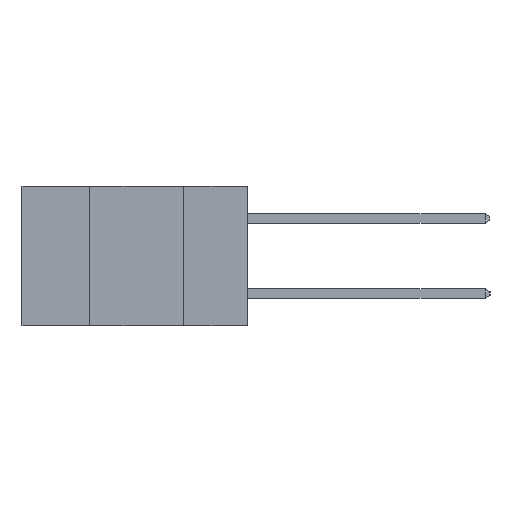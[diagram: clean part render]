
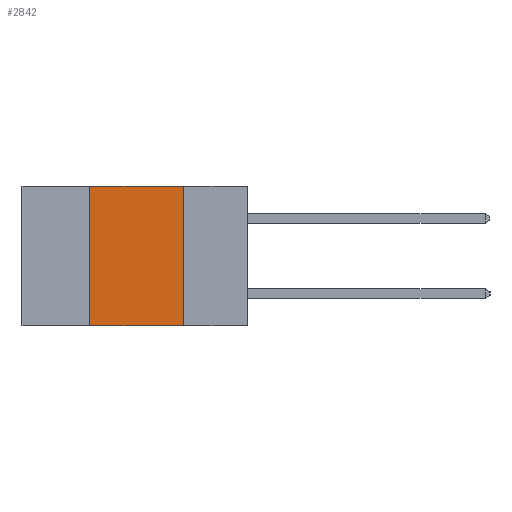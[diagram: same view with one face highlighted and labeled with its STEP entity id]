
A CAD part, left-side view. The second image highlights one B-rep face of the part: STEP entity #2842.
In plain terms, the highlighted planar face has unit normal (-1, 0, 0).
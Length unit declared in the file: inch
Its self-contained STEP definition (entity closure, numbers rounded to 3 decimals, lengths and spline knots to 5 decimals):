
#142 = VECTOR ( 'NONE', #5991, 39.37008 ) ;
#440 = VECTOR ( 'NONE', #12052, 39.37008 ) ;
#1023 = VERTEX_POINT ( 'NONE', #17797 ) ;
#1209 = DIRECTION ( 'NONE',  ( 0., 0., -1. ) ) ;
#1297 = ORIENTED_EDGE ( 'NONE', *, *, #7673, .F. ) ;
#1351 = DIRECTION ( 'NONE',  ( 1., 0., 0. ) ) ;
#1545 = CARTESIAN_POINT ( 'NONE',  ( 0., 0.6, 0. ) ) ;
#1563 = PLANE ( 'NONE',  #12263 ) ;
#1833 = DIRECTION ( 'NONE',  ( 0., 0., 1. ) ) ;
#2842 = ADVANCED_FACE ( 'NONE', ( #9797 ), #1563, .F. ) ;
#2992 = VERTEX_POINT ( 'NONE', #19221 ) ;
#3290 = CARTESIAN_POINT ( 'NONE',  ( 0., 0.42, -0.37 ) ) ;
#3677 = DIRECTION ( 'NONE',  ( 0., 0., -1. ) ) ;
#4382 = EDGE_CURVE ( 'NONE', #12080, #2992, #7931, .T. ) ;
#5432 = CARTESIAN_POINT ( 'NONE',  ( 0., 0.17, -0.37 ) ) ;
#5991 = DIRECTION ( 'NONE',  ( 0., -1., 0. ) ) ;
#6108 = CARTESIAN_POINT ( 'NONE',  ( 0., 0.6, -0.37 ) ) ;
#7249 = LINE ( 'NONE', #19880, #20159 ) ;
#7673 = EDGE_CURVE ( 'NONE', #2992, #1023, #9186, .T. ) ;
#7931 = LINE ( 'NONE', #3290, #19820 ) ;
#9010 = ORIENTED_EDGE ( 'NONE', *, *, #20681, .F. ) ;
#9186 = LINE ( 'NONE', #12073, #440 ) ;
#9338 = ORIENTED_EDGE ( 'NONE', *, *, #4382, .F. ) ;
#9460 = EDGE_CURVE ( 'NONE', #12080, #16480, #9913, .T. ) ;
#9797 = FACE_OUTER_BOUND ( 'NONE', #20126, .T. ) ;
#9876 = ORIENTED_EDGE ( 'NONE', *, *, #9460, .T. ) ;
#9913 = LINE ( 'NONE', #6108, #142 ) ;
#12052 = DIRECTION ( 'NONE',  ( 0., -1., 0. ) ) ;
#12073 = CARTESIAN_POINT ( 'NONE',  ( 0., 0.6, 0. ) ) ;
#12080 = VERTEX_POINT ( 'NONE', #17121 ) ;
#12263 = AXIS2_PLACEMENT_3D ( 'NONE', #1545, #1351, #1209 ) ;
#16480 = VERTEX_POINT ( 'NONE', #5432 ) ;
#17121 = CARTESIAN_POINT ( 'NONE',  ( 0., 0.42, -0.37 ) ) ;
#17797 = CARTESIAN_POINT ( 'NONE',  ( 0., 0.17, 0. ) ) ;
#19221 = CARTESIAN_POINT ( 'NONE',  ( 0., 0.42, 0. ) ) ;
#19820 = VECTOR ( 'NONE', #1833, 39.37008 ) ;
#19880 = CARTESIAN_POINT ( 'NONE',  ( 0., 0.17, -0.37 ) ) ;
#20126 = EDGE_LOOP ( 'NONE', ( #9010, #1297, #9338, #9876 ) ) ;
#20159 = VECTOR ( 'NONE', #3677, 39.37008 ) ;
#20681 = EDGE_CURVE ( 'NONE', #1023, #16480, #7249, .T. ) ;
